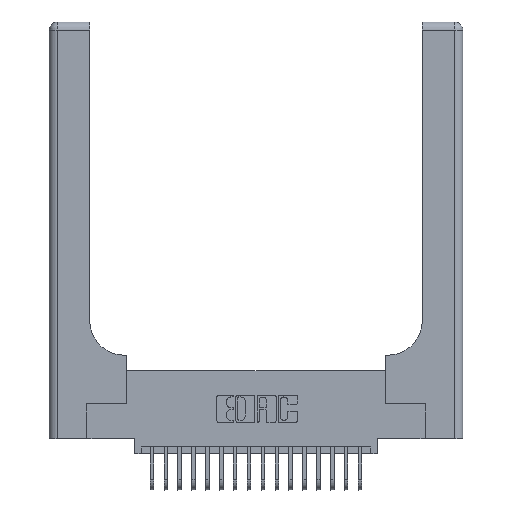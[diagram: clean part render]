
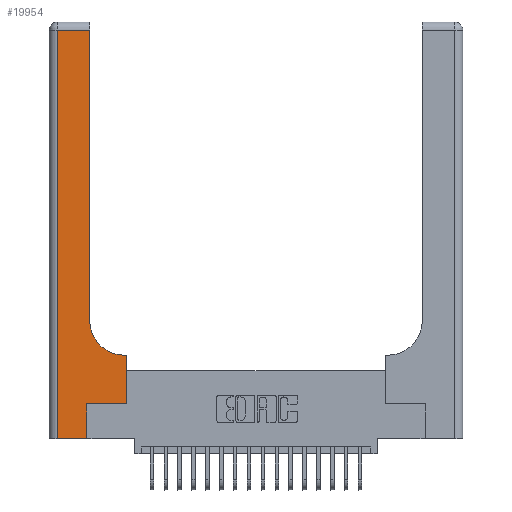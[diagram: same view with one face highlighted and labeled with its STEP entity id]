
A CAD part, top view. The second image highlights one B-rep face of the part: STEP entity #19954.
In plain terms, the highlighted planar face has unit normal (0, 0, 1).
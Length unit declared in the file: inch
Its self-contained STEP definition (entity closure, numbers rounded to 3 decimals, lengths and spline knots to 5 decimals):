
#133 = CARTESIAN_POINT ( 'NONE',  ( 0.269, 0., 0.37 ) ) ;
#453 = LINE ( 'NONE', #9774, #5762 ) ;
#823 = DIRECTION ( 'NONE',  ( 1., 0., 0. ) ) ;
#944 = EDGE_CURVE ( 'NONE', #15201, #13297, #453, .T. ) ;
#1000 = EDGE_CURVE ( 'NONE', #13950, #1063, #5227, .T. ) ;
#1063 = VERTEX_POINT ( 'NONE', #13644 ) ;
#1115 = ORIENTED_EDGE ( 'NONE', *, *, #1000, .T. ) ;
#2091 = CARTESIAN_POINT ( 'NONE',  ( 0.269, 0., 0.37 ) ) ;
#2326 = CARTESIAN_POINT ( 'NONE',  ( 0.5415, 0.85, 0.37 ) ) ;
#2672 = CARTESIAN_POINT ( 'NONE',  ( 0.2915, 0.6, 0.37 ) ) ;
#2831 = CARTESIAN_POINT ( 'NONE',  ( 0., 2.94, 0.37 ) ) ;
#2934 = ORIENTED_EDGE ( 'NONE', *, *, #17236, .T. ) ;
#3072 = CARTESIAN_POINT ( 'NONE',  ( 0.2915, 2.94, 0.37 ) ) ;
#3252 = EDGE_CURVE ( 'NONE', #13297, #13950, #8483, .T. ) ;
#4017 = CARTESIAN_POINT ( 'NONE',  ( 0.2915, 0.85, 0.37 ) ) ;
#4581 = DIRECTION ( 'NONE',  ( -1., 0., 0. ) ) ;
#4623 = DIRECTION ( 'NONE',  ( -1., 0., 0. ) ) ;
#5227 = LINE ( 'NONE', #6665, #17158 ) ;
#5697 = EDGE_CURVE ( 'NONE', #19637, #13146, #11250, .T. ) ;
#5762 = VECTOR ( 'NONE', #823, 39.37008 ) ;
#5963 = DIRECTION ( 'NONE',  ( 0., 0., -1. ) ) ;
#6403 = ORIENTED_EDGE ( 'NONE', *, *, #21140, .T. ) ;
#6610 = CARTESIAN_POINT ( 'NONE',  ( 0.269, 0.25, 0.37 ) ) ;
#6665 = CARTESIAN_POINT ( 'NONE',  ( 0.269, 0.25, 0.37 ) ) ;
#6697 = VERTEX_POINT ( 'NONE', #3072 ) ;
#6988 = DIRECTION ( 'NONE',  ( 0., 1., 0. ) ) ;
#7049 = VECTOR ( 'NONE', #6988, 39.37008 ) ;
#7782 = VECTOR ( 'NONE', #8287, 39.37008 ) ;
#8177 = ORIENTED_EDGE ( 'NONE', *, *, #13172, .T. ) ;
#8287 = DIRECTION ( 'NONE',  ( 0., -1., 0. ) ) ;
#8483 = LINE ( 'NONE', #2091, #15162 ) ;
#8606 = LINE ( 'NONE', #20832, #21101 ) ;
#9380 = FACE_OUTER_BOUND ( 'NONE', #13176, .T. ) ;
#9774 = CARTESIAN_POINT ( 'NONE',  ( 0., 0., 0.37 ) ) ;
#10181 = DIRECTION ( 'NONE',  ( 0., 1., 0. ) ) ;
#10235 = CARTESIAN_POINT ( 'NONE',  ( 0.5585, 0.6, 0.37 ) ) ;
#10495 = CARTESIAN_POINT ( 'NONE',  ( 0.2915, 3., 0.37 ) ) ;
#10768 = DIRECTION ( 'NONE',  ( -1., 0., 0. ) ) ;
#11250 = LINE ( 'NONE', #2672, #18187 ) ;
#11318 = CARTESIAN_POINT ( 'NONE',  ( 0.06, 0., 0.37 ) ) ;
#11505 = CARTESIAN_POINT ( 'NONE',  ( 0.5415, 0.6, 0.37 ) ) ;
#13146 = VERTEX_POINT ( 'NONE', #11505 ) ;
#13172 = EDGE_CURVE ( 'NONE', #13146, #22329, #17848, .T. ) ;
#13176 = EDGE_LOOP ( 'NONE', ( #6403, #2934, #14957, #16171, #22639, #1115, #21374, #16235, #8177 ) ) ;
#13297 = VERTEX_POINT ( 'NONE', #133 ) ;
#13644 = CARTESIAN_POINT ( 'NONE',  ( 0.5585, 0.25, 0.37 ) ) ;
#13742 = VERTEX_POINT ( 'NONE', #18409 ) ;
#13950 = VERTEX_POINT ( 'NONE', #6610 ) ;
#13995 = DIRECTION ( 'NONE',  ( 1., 0., 0. ) ) ;
#14496 = DIRECTION ( 'NONE',  ( 0., 0., -1. ) ) ;
#14957 = ORIENTED_EDGE ( 'NONE', *, *, #18572, .T. ) ;
#15162 = VECTOR ( 'NONE', #15211, 39.37008 ) ;
#15201 = VERTEX_POINT ( 'NONE', #11318 ) ;
#15211 = DIRECTION ( 'NONE',  ( 0., 1., 0. ) ) ;
#15754 = CARTESIAN_POINT ( 'NONE',  ( 0.06, 3., 0.37 ) ) ;
#16027 = DIRECTION ( 'NONE',  ( 1., 0., 0. ) ) ;
#16171 = ORIENTED_EDGE ( 'NONE', *, *, #944, .T. ) ;
#16235 = ORIENTED_EDGE ( 'NONE', *, *, #5697, .T. ) ;
#16913 = AXIS2_PLACEMENT_3D ( 'NONE', #2326, #5963, #16027 ) ;
#17158 = VECTOR ( 'NONE', #13995, 39.37008 ) ;
#17236 = EDGE_CURVE ( 'NONE', #6697, #13742, #20892, .T. ) ;
#17848 = CIRCLE ( 'NONE', #16913, 0.25 ) ;
#17974 = PLANE ( 'NONE',  #21934 ) ;
#18187 = VECTOR ( 'NONE', #4581, 39.37008 ) ;
#18409 = CARTESIAN_POINT ( 'NONE',  ( 0.06, 2.94, 0.37 ) ) ;
#18572 = EDGE_CURVE ( 'NONE', #13742, #15201, #20289, .T. ) ;
#19091 = EDGE_CURVE ( 'NONE', #1063, #19637, #8606, .T. ) ;
#19215 = VECTOR ( 'NONE', #4623, 39.37008 ) ;
#19637 = VERTEX_POINT ( 'NONE', #10235 ) ;
#19954 = ADVANCED_FACE ( 'NONE', ( #9380 ), #17974, .F. ) ;
#20289 = LINE ( 'NONE', #15754, #7782 ) ;
#20832 = CARTESIAN_POINT ( 'NONE',  ( 0.5585, 0.25, 0.37 ) ) ;
#20892 = LINE ( 'NONE', #2831, #19215 ) ;
#21101 = VECTOR ( 'NONE', #10181, 39.37008 ) ;
#21140 = EDGE_CURVE ( 'NONE', #22329, #6697, #21772, .T. ) ;
#21374 = ORIENTED_EDGE ( 'NONE', *, *, #19091, .T. ) ;
#21549 = CARTESIAN_POINT ( 'NONE',  ( 0., 3., 0.37 ) ) ;
#21772 = LINE ( 'NONE', #10495, #7049 ) ;
#21934 = AXIS2_PLACEMENT_3D ( 'NONE', #21549, #14496, #10768 ) ;
#22329 = VERTEX_POINT ( 'NONE', #4017 ) ;
#22639 = ORIENTED_EDGE ( 'NONE', *, *, #3252, .T. ) ;
